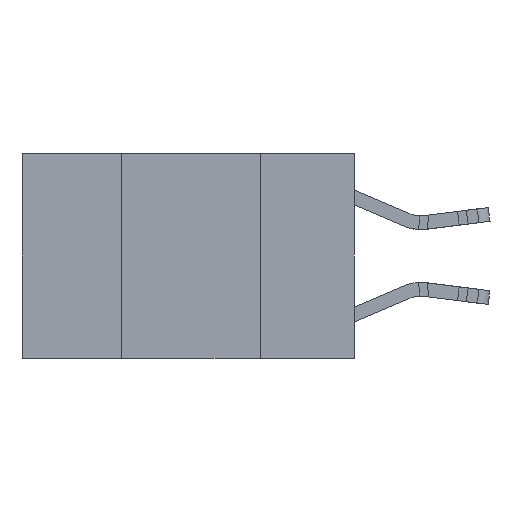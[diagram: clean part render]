
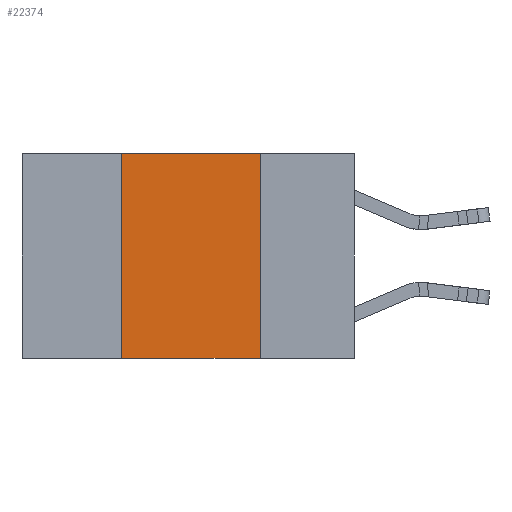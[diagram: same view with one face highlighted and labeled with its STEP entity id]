
A CAD part, left-side view. The second image highlights one B-rep face of the part: STEP entity #22374.
In plain terms, the highlighted planar face has unit normal (-1, 0, 0).
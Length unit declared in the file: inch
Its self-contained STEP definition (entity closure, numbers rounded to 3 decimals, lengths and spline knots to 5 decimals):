
#623 = VERTEX_POINT ( 'NONE', #10480 ) ;
#1436 = VECTOR ( 'NONE', #27509, 39.37008 ) ;
#2192 = CARTESIAN_POINT ( 'NONE',  ( 0., 0.17, -0.37 ) ) ;
#2286 = VECTOR ( 'NONE', #27967, 39.37008 ) ;
#4222 = AXIS2_PLACEMENT_3D ( 'NONE', #13623, #27064, #13722 ) ;
#5202 = CARTESIAN_POINT ( 'NONE',  ( 0., 0.17, 0. ) ) ;
#5467 = ORIENTED_EDGE ( 'NONE', *, *, #11719, .F. ) ;
#6180 = ORIENTED_EDGE ( 'NONE', *, *, #17042, .T. ) ;
#6898 = VECTOR ( 'NONE', #26500, 39.37008 ) ;
#8223 = VERTEX_POINT ( 'NONE', #15238 ) ;
#9261 = EDGE_CURVE ( 'NONE', #623, #22274, #14052, .T. ) ;
#10480 = CARTESIAN_POINT ( 'NONE',  ( 0., 0.17, 0. ) ) ;
#10884 = CARTESIAN_POINT ( 'NONE',  ( 0., 0.6, -0.37 ) ) ;
#11719 = EDGE_CURVE ( 'NONE', #28240, #623, #24360, .T. ) ;
#12158 = CARTESIAN_POINT ( 'NONE',  ( 0., 0.6, 0. ) ) ;
#12809 = LINE ( 'NONE', #10884, #6898 ) ;
#13623 = CARTESIAN_POINT ( 'NONE',  ( 0., 0.6, 0. ) ) ;
#13722 = DIRECTION ( 'NONE',  ( 0., 0., -1. ) ) ;
#14052 = LINE ( 'NONE', #5202, #1436 ) ;
#14648 = CARTESIAN_POINT ( 'NONE',  ( 0., 0.42, 0. ) ) ;
#15238 = CARTESIAN_POINT ( 'NONE',  ( 0., 0.42, -0.37 ) ) ;
#17042 = EDGE_CURVE ( 'NONE', #8223, #22274, #12809, .T. ) ;
#17500 = EDGE_LOOP ( 'NONE', ( #22578, #5467, #23269, #6180 ) ) ;
#18118 = FACE_OUTER_BOUND ( 'NONE', #17500, .T. ) ;
#18474 = VECTOR ( 'NONE', #21203, 39.37008 ) ;
#21203 = DIRECTION ( 'NONE',  ( 0., -1., 0. ) ) ;
#22274 = VERTEX_POINT ( 'NONE', #2192 ) ;
#22374 = ADVANCED_FACE ( 'NONE', ( #18118 ), #24830, .F. ) ;
#22578 = ORIENTED_EDGE ( 'NONE', *, *, #9261, .F. ) ;
#23269 = ORIENTED_EDGE ( 'NONE', *, *, #23881, .F. ) ;
#23881 = EDGE_CURVE ( 'NONE', #8223, #28240, #26033, .T. ) ;
#24360 = LINE ( 'NONE', #12158, #18474 ) ;
#24830 = PLANE ( 'NONE',  #4222 ) ;
#26033 = LINE ( 'NONE', #14648, #2286 ) ;
#26500 = DIRECTION ( 'NONE',  ( 0., -1., 0. ) ) ;
#26621 = CARTESIAN_POINT ( 'NONE',  ( 0., 0.42, 0. ) ) ;
#27064 = DIRECTION ( 'NONE',  ( 1., 0., 0. ) ) ;
#27509 = DIRECTION ( 'NONE',  ( 0., 0., -1. ) ) ;
#27967 = DIRECTION ( 'NONE',  ( 0., 0., 1. ) ) ;
#28240 = VERTEX_POINT ( 'NONE', #26621 ) ;
